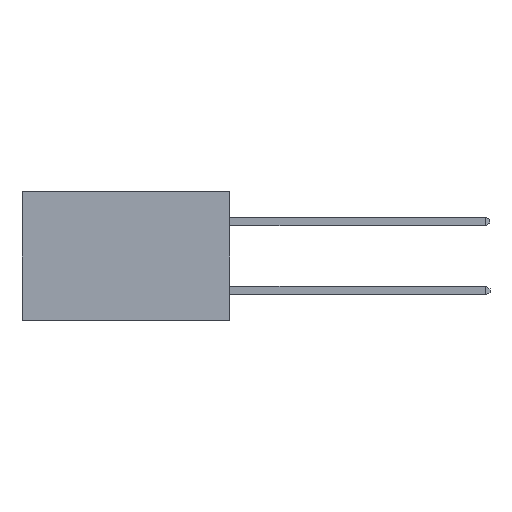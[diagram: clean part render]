
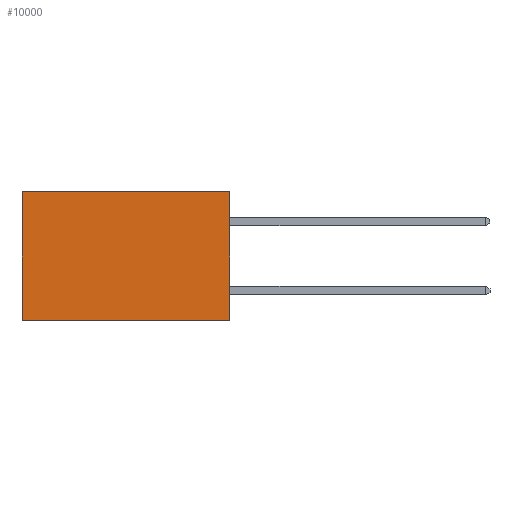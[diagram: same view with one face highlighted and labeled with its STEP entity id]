
A CAD part, left-side view. The second image highlights one B-rep face of the part: STEP entity #10000.
In plain terms, the highlighted planar face has unit normal (-1, 0, 0).
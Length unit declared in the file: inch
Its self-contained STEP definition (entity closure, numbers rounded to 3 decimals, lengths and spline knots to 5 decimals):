
#67 = CARTESIAN_POINT ( 'NONE',  ( 0.2615, 0.6, -0.37 ) ) ;
#339 = DIRECTION ( 'NONE',  ( 0., 0., -1. ) ) ;
#820 = VECTOR ( 'NONE', #6214, 39.37008 ) ;
#1267 = DIRECTION ( 'NONE',  ( 0., 0., -1. ) ) ;
#1459 = LINE ( 'NONE', #67, #3538 ) ;
#1752 = DIRECTION ( 'NONE',  ( 1., 0., 0. ) ) ;
#1941 = CARTESIAN_POINT ( 'NONE',  ( 0.2615, 0., -0.37 ) ) ;
#2170 = PLANE ( 'NONE',  #10872 ) ;
#2295 = VECTOR ( 'NONE', #3145, 39.37008 ) ;
#2576 = LINE ( 'NONE', #3124, #2295 ) ;
#2619 = EDGE_CURVE ( 'NONE', #10656, #2682, #1459, .T. ) ;
#2682 = VERTEX_POINT ( 'NONE', #6180 ) ;
#3124 = CARTESIAN_POINT ( 'NONE',  ( 0.2615, 0., 0. ) ) ;
#3145 = DIRECTION ( 'NONE',  ( 0., 1., 0. ) ) ;
#3256 = LINE ( 'NONE', #6334, #820 ) ;
#3538 = VECTOR ( 'NONE', #339, 39.37008 ) ;
#3714 = VECTOR ( 'NONE', #6057, 39.37008 ) ;
#3734 = CARTESIAN_POINT ( 'NONE',  ( 0.2615, 0., -0.37 ) ) ;
#5184 = ORIENTED_EDGE ( 'NONE', *, *, #2619, .T. ) ;
#6057 = DIRECTION ( 'NONE',  ( 0., 1., 0. ) ) ;
#6058 = ORIENTED_EDGE ( 'NONE', *, *, #10965, .T. ) ;
#6180 = CARTESIAN_POINT ( 'NONE',  ( 0.2615, 0.6, -0.37 ) ) ;
#6214 = DIRECTION ( 'NONE',  ( 0., 0., -1. ) ) ;
#6228 = CARTESIAN_POINT ( 'NONE',  ( 0.2615, 0.6, 0. ) ) ;
#6334 = CARTESIAN_POINT ( 'NONE',  ( 0.2615, 0., -0.37 ) ) ;
#6384 = LINE ( 'NONE', #3734, #3714 ) ;
#6900 = VERTEX_POINT ( 'NONE', #9674 ) ;
#8932 = EDGE_CURVE ( 'NONE', #6900, #2682, #6384, .T. ) ;
#9127 = FACE_OUTER_BOUND ( 'NONE', #10023, .T. ) ;
#9414 = CARTESIAN_POINT ( 'NONE',  ( 0.2615, 0., 0. ) ) ;
#9674 = CARTESIAN_POINT ( 'NONE',  ( 0.2615, 0., -0.37 ) ) ;
#10000 = ADVANCED_FACE ( 'NONE', ( #9127 ), #2170, .F. ) ;
#10023 = EDGE_LOOP ( 'NONE', ( #5184, #10992, #10777, #6058 ) ) ;
#10302 = VERTEX_POINT ( 'NONE', #9414 ) ;
#10654 = EDGE_CURVE ( 'NONE', #10302, #6900, #3256, .T. ) ;
#10656 = VERTEX_POINT ( 'NONE', #6228 ) ;
#10777 = ORIENTED_EDGE ( 'NONE', *, *, #10654, .F. ) ;
#10872 = AXIS2_PLACEMENT_3D ( 'NONE', #1941, #1752, #1267 ) ;
#10965 = EDGE_CURVE ( 'NONE', #10302, #10656, #2576, .T. ) ;
#10992 = ORIENTED_EDGE ( 'NONE', *, *, #8932, .F. ) ;
